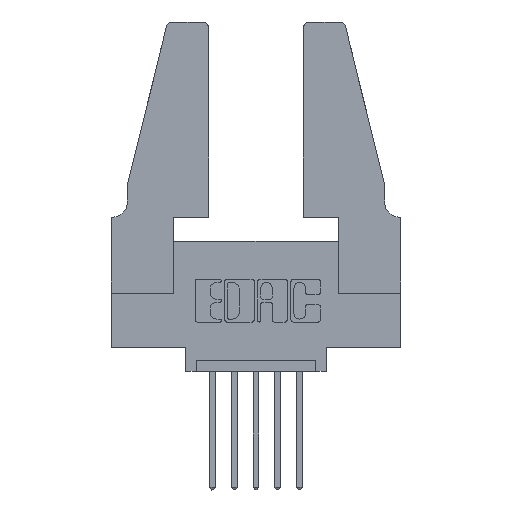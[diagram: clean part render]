
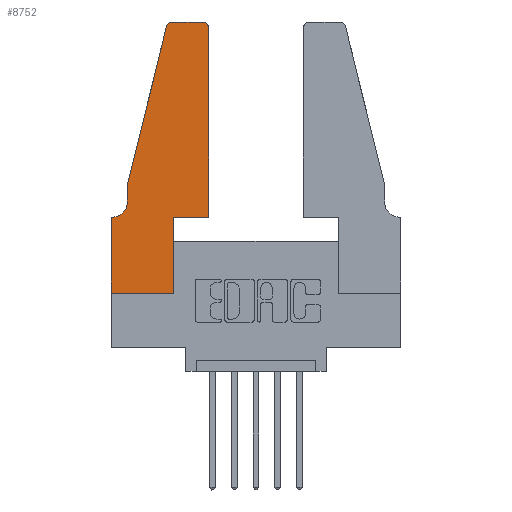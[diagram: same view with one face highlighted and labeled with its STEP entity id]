
A CAD part, top view. The second image highlights one B-rep face of the part: STEP entity #8752.
In plain terms, the highlighted planar face has unit normal (0, 0, 1).
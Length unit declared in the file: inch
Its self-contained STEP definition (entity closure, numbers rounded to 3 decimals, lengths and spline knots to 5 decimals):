
#61 = VECTOR ( 'NONE', #5453, 39.37008 ) ;
#90 = VECTOR ( 'NONE', #626, 39.37008 ) ;
#298 = EDGE_CURVE ( 'NONE', #10809, #10760, #11074, .T. ) ;
#365 = LINE ( 'NONE', #9460, #6909 ) ;
#395 = CARTESIAN_POINT ( 'NONE',  ( 0.4505, 1.22, 0.37 ) ) ;
#405 = AXIS2_PLACEMENT_3D ( 'NONE', #8813, #2052, #3791 ) ;
#626 = DIRECTION ( 'NONE',  ( 0., 1., 0. ) ) ;
#637 = CARTESIAN_POINT ( 'NONE',  ( 0.2865, 0.35, 0.37 ) ) ;
#719 = CARTESIAN_POINT ( 'NONE',  ( 0.2865, 0., 0.37 ) ) ;
#822 = CIRCLE ( 'NONE', #4211, 0.03 ) ;
#932 = LINE ( 'NONE', #5086, #6799 ) ;
#1048 = LINE ( 'NONE', #4091, #90 ) ;
#1087 = CARTESIAN_POINT ( 'NONE',  ( 0.0055, 0.35, 0.37 ) ) ;
#1138 = CARTESIAN_POINT ( 'NONE',  ( 0.4505, 0.35, 0.37 ) ) ;
#1234 = VERTEX_POINT ( 'NONE', #9413 ) ;
#1276 = VERTEX_POINT ( 'NONE', #7914 ) ;
#1294 = EDGE_CURVE ( 'NONE', #6485, #3760, #1889, .T. ) ;
#1412 = ORIENTED_EDGE ( 'NONE', *, *, #8224, .T. ) ;
#1420 = DIRECTION ( 'NONE',  ( 0., 0., 1. ) ) ;
#1477 = VECTOR ( 'NONE', #3064, 39.37008 ) ;
#1522 = VERTEX_POINT ( 'NONE', #4077 ) ;
#1568 = ORIENTED_EDGE ( 'NONE', *, *, #8477, .T. ) ;
#1889 = LINE ( 'NONE', #2823, #2298 ) ;
#2052 = DIRECTION ( 'NONE',  ( 0., 0., -1. ) ) ;
#2104 = CARTESIAN_POINT ( 'NONE',  ( 0.0755, 0.35, 0.37 ) ) ;
#2154 = EDGE_CURVE ( 'NONE', #10760, #4663, #6510, .T. ) ;
#2219 = PLANE ( 'NONE',  #9175 ) ;
#2292 = DIRECTION ( 'NONE',  ( 1., 0., 0. ) ) ;
#2294 = AXIS2_PLACEMENT_3D ( 'NONE', #5687, #1420, #7370 ) ;
#2298 = VECTOR ( 'NONE', #8773, 39.37008 ) ;
#2823 = CARTESIAN_POINT ( 'NONE',  ( 0.2605, 1.25, 0.37 ) ) ;
#3064 = DIRECTION ( 'NONE',  ( -1., 0., 0. ) ) ;
#3097 = CARTESIAN_POINT ( 'NONE',  ( 0., 0.35, 0.37 ) ) ;
#3496 = EDGE_CURVE ( 'NONE', #7372, #10809, #7696, .T. ) ;
#3619 = VECTOR ( 'NONE', #5491, 39.37008 ) ;
#3760 = VERTEX_POINT ( 'NONE', #10469 ) ;
#3791 = DIRECTION ( 'NONE',  ( -1., 0., 0. ) ) ;
#3829 = DIRECTION ( 'NONE',  ( 1., 0., 0. ) ) ;
#4077 = CARTESIAN_POINT ( 'NONE',  ( 0.4505, 0.35, 0.37 ) ) ;
#4091 = CARTESIAN_POINT ( 'NONE',  ( 0.4505, 0.35, 0.37 ) ) ;
#4118 = CARTESIAN_POINT ( 'NONE',  ( 0.2865, 0.35, 0.37 ) ) ;
#4211 = AXIS2_PLACEMENT_3D ( 'NONE', #7300, #8185, #10717 ) ;
#4246 = ORIENTED_EDGE ( 'NONE', *, *, #3496, .T. ) ;
#4663 = VERTEX_POINT ( 'NONE', #4118 ) ;
#4731 = CARTESIAN_POINT ( 'NONE',  ( 0., 0., 0.37 ) ) ;
#5052 = VECTOR ( 'NONE', #9189, 39.37008 ) ;
#5086 = CARTESIAN_POINT ( 'NONE',  ( 0.0755, 0.5, 0.37 ) ) ;
#5453 = DIRECTION ( 'NONE',  ( 0., -1., 0. ) ) ;
#5491 = DIRECTION ( 'NONE',  ( 1., 0., 0. ) ) ;
#5568 = VERTEX_POINT ( 'NONE', #395 ) ;
#5640 = EDGE_CURVE ( 'NONE', #5568, #6485, #8065, .T. ) ;
#5687 = CARTESIAN_POINT ( 'NONE',  ( 0.4205, 1.22, 0.37 ) ) ;
#5762 = CARTESIAN_POINT ( 'NONE',  ( 0., 0., 0.37 ) ) ;
#5900 = ORIENTED_EDGE ( 'NONE', *, *, #2154, .T. ) ;
#5902 = EDGE_CURVE ( 'NONE', #3760, #6942, #822, .T. ) ;
#5988 = LINE ( 'NONE', #2104, #1477 ) ;
#6004 = DIRECTION ( 'NONE',  ( 0., -1., 0. ) ) ;
#6088 = CARTESIAN_POINT ( 'NONE',  ( 0.4205, 1.25, 0.37 ) ) ;
#6155 = DIRECTION ( 'NONE',  ( -0.239, -0.971, 0. ) ) ;
#6485 = VERTEX_POINT ( 'NONE', #6088 ) ;
#6510 = LINE ( 'NONE', #637, #5052 ) ;
#6734 = VERTEX_POINT ( 'NONE', #1087 ) ;
#6799 = VECTOR ( 'NONE', #6004, 39.37008 ) ;
#6909 = VECTOR ( 'NONE', #6155, 39.37008 ) ;
#6942 = VERTEX_POINT ( 'NONE', #9604 ) ;
#7300 = CARTESIAN_POINT ( 'NONE',  ( 0.284, 1.22, 0.37 ) ) ;
#7347 = VECTOR ( 'NONE', #2292, 39.37008 ) ;
#7363 = ORIENTED_EDGE ( 'NONE', *, *, #5902, .T. ) ;
#7367 = EDGE_CURVE ( 'NONE', #1276, #1234, #932, .T. ) ;
#7370 = DIRECTION ( 'NONE',  ( 1., 0., 0. ) ) ;
#7372 = VERTEX_POINT ( 'NONE', #10262 ) ;
#7612 = EDGE_CURVE ( 'NONE', #1234, #6734, #10795, .T. ) ;
#7696 = LINE ( 'NONE', #4731, #61 ) ;
#7914 = CARTESIAN_POINT ( 'NONE',  ( 0.0755, 0.5, 0.37 ) ) ;
#8065 = CIRCLE ( 'NONE', #2294, 0.03 ) ;
#8185 = DIRECTION ( 'NONE',  ( 0., 0., 1. ) ) ;
#8224 = EDGE_CURVE ( 'NONE', #1522, #5568, #1048, .T. ) ;
#8274 = ORIENTED_EDGE ( 'NONE', *, *, #5640, .T. ) ;
#8477 = EDGE_CURVE ( 'NONE', #6942, #1276, #365, .T. ) ;
#8752 = ADVANCED_FACE ( 'NONE', ( #10773 ), #2219, .T. ) ;
#8773 = DIRECTION ( 'NONE',  ( -1., 0., 0. ) ) ;
#8813 = CARTESIAN_POINT ( 'NONE',  ( 0.0055, 0.42, 0.37 ) ) ;
#8923 = EDGE_LOOP ( 'NONE', ( #10053, #7363, #1568, #10547, #9981, #10491, #4246, #9130, #5900, #9041, #1412, #8274 ) ) ;
#9041 = ORIENTED_EDGE ( 'NONE', *, *, #10991, .T. ) ;
#9052 = DIRECTION ( 'NONE',  ( 0., 0., 1. ) ) ;
#9130 = ORIENTED_EDGE ( 'NONE', *, *, #298, .T. ) ;
#9175 = AXIS2_PLACEMENT_3D ( 'NONE', #3097, #9052, #3829 ) ;
#9189 = DIRECTION ( 'NONE',  ( 0., 1., 0. ) ) ;
#9413 = CARTESIAN_POINT ( 'NONE',  ( 0.0755, 0.42, 0.37 ) ) ;
#9460 = CARTESIAN_POINT ( 'NONE',  ( 0.0755, 0.5, 0.37 ) ) ;
#9604 = CARTESIAN_POINT ( 'NONE',  ( 0.25487, 1.22718, 0.37 ) ) ;
#9981 = ORIENTED_EDGE ( 'NONE', *, *, #7612, .T. ) ;
#10053 = ORIENTED_EDGE ( 'NONE', *, *, #1294, .T. ) ;
#10247 = LINE ( 'NONE', #1138, #3619 ) ;
#10262 = CARTESIAN_POINT ( 'NONE',  ( 0., 0.35, 0.37 ) ) ;
#10312 = CARTESIAN_POINT ( 'NONE',  ( 0., 0., 0.37 ) ) ;
#10455 = EDGE_CURVE ( 'NONE', #6734, #7372, #5988, .T. ) ;
#10469 = CARTESIAN_POINT ( 'NONE',  ( 0.284, 1.25, 0.37 ) ) ;
#10491 = ORIENTED_EDGE ( 'NONE', *, *, #10455, .T. ) ;
#10547 = ORIENTED_EDGE ( 'NONE', *, *, #7367, .T. ) ;
#10717 = DIRECTION ( 'NONE',  ( 1., 0., 0. ) ) ;
#10760 = VERTEX_POINT ( 'NONE', #719 ) ;
#10773 = FACE_OUTER_BOUND ( 'NONE', #8923, .T. ) ;
#10795 = CIRCLE ( 'NONE', #405, 0.07 ) ;
#10809 = VERTEX_POINT ( 'NONE', #10312 ) ;
#10991 = EDGE_CURVE ( 'NONE', #4663, #1522, #10247, .T. ) ;
#11074 = LINE ( 'NONE', #5762, #7347 ) ;
